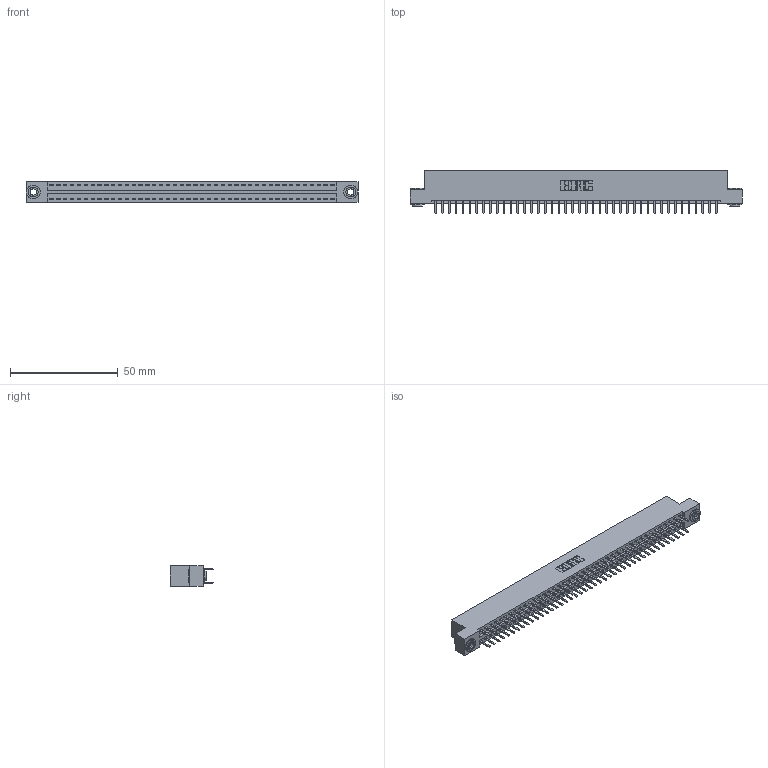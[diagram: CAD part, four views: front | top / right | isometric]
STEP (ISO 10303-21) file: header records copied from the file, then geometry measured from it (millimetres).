
FILE_DESCRIPTION (( 'STEP AP203' ), '1' );
FILE_NAME ('396-084-520-203.STEP', '2019-10-30T23:47:11', ( '' ), ( '' ), 'SwSTEP 2.0', 'SolidWorks 2016', '' );
FILE_SCHEMA (( 'CONFIG_CONTROL_DESIGN' ));
Length unit declared in the file: inch
Products named in the file (4): 396-084-520-203; 346 Part_Flush Mounting Lugs - 0.156 Dia-TH; 345-250-002_345-250-002-102; 345-292-001_345-293-120
Assembly tree (87 placements, depth 2):
  396-084-520-203
    346 Part_Flush Mounting Lugs - 0.156 Dia-TH
    345-292-001_345-293-120  x84
    345-250-002_345-250-002-102  x2
Bounding box: 153.92 x 20.02 x 9.4 mm (x, y, z)
Volume: 14992 mm3; surface area: 20735.1 mm2
Topology: 87 solids, 87 shells, 4864 faces, 14097 edges, 9170 vertices
Faces by surface type: plane 3194, cylinder 1662, cone 8
Entity records: 28174 total; most frequent: CARTESIAN_POINT 4631, ORIENTED_EDGE 4546, DIRECTION 4151, EDGE_CURVE 2273, LINE 1945, VECTOR 1945, VERTEX_POINT 1510, AXIS2_PLACEMENT_3D 1103
